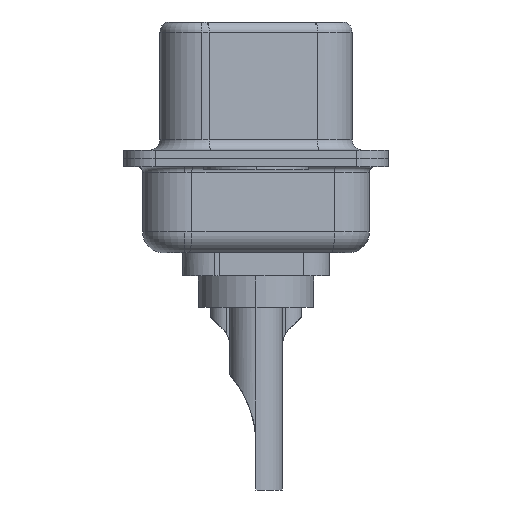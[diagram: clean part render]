
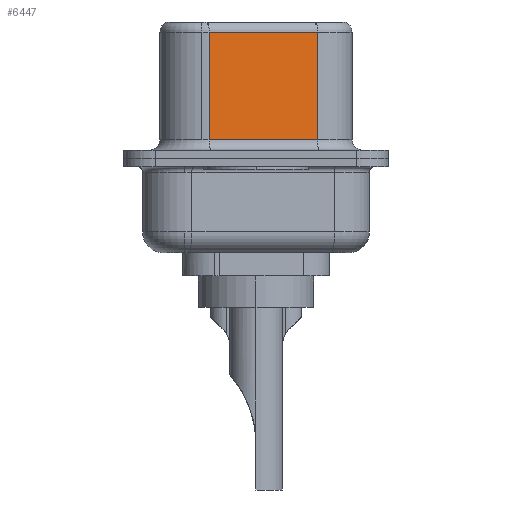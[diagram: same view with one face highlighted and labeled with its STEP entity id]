
A CAD part, left-side view. The second image highlights one B-rep face of the part: STEP entity #6447.
In plain terms, the highlighted planar face has unit normal (-0.985, -0.174, 0).
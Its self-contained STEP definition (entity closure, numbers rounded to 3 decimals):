
#517 = DIRECTION ( 'NONE',  ( 0.985, 0.174, 0. ) ) ;
#656 = DIRECTION ( 'NONE',  ( 0.174, -0.985, 0. ) ) ;
#715 = VECTOR ( 'NONE', #656, 1000. ) ;
#895 = EDGE_CURVE ( 'NONE', #2438, #12304, #14411, .T. ) ;
#1305 = AXIS2_PLACEMENT_3D ( 'NONE', #20225, #517, #16758 ) ;
#2438 = VERTEX_POINT ( 'NONE', #20954 ) ;
#2993 = CARTESIAN_POINT ( 'NONE',  ( 3.67, 2.233, 0.9 ) ) ;
#3220 = ORIENTED_EDGE ( 'NONE', *, *, #12690, .F. ) ;
#3221 = VERTEX_POINT ( 'NONE', #16325 ) ;
#3273 = VECTOR ( 'NONE', #15932, 1000. ) ;
#3303 = DIRECTION ( 'NONE',  ( -0.174, 0.985, 0. ) ) ;
#3773 = EDGE_CURVE ( 'NONE', #12304, #20291, #18393, .T. ) ;
#5034 = LINE ( 'NONE', #10408, #715 ) ;
#6155 = CARTESIAN_POINT ( 'NONE',  ( 4.58, -2.927, 6.52 ) ) ;
#6447 = ADVANCED_FACE ( 'NONE', ( #16624 ), #12303, .F. ) ;
#6517 = ORIENTED_EDGE ( 'NONE', *, *, #895, .T. ) ;
#9609 = ORIENTED_EDGE ( 'NONE', *, *, #3773, .T. ) ;
#9735 = VECTOR ( 'NONE', #19450, 1000. ) ;
#9785 = CARTESIAN_POINT ( 'NONE',  ( 3.67, 2.233, 6.02 ) ) ;
#9902 = ORIENTED_EDGE ( 'NONE', *, *, #18076, .T. ) ;
#10408 = CARTESIAN_POINT ( 'NONE',  ( 4.58, -2.927, 0.9 ) ) ;
#10554 = VECTOR ( 'NONE', #3303, 1000. ) ;
#11440 = LINE ( 'NONE', #6155, #3273 ) ;
#12303 = PLANE ( 'NONE',  #1305 ) ;
#12304 = VERTEX_POINT ( 'NONE', #9785 ) ;
#12690 = EDGE_CURVE ( 'NONE', #2438, #3221, #11440, .T. ) ;
#13580 = CARTESIAN_POINT ( 'NONE',  ( 4.58, -2.927, 6.02 ) ) ;
#13636 = CARTESIAN_POINT ( 'NONE',  ( 3.67, 2.233, 6.52 ) ) ;
#14411 = LINE ( 'NONE', #13580, #10554 ) ;
#15401 = EDGE_LOOP ( 'NONE', ( #3220, #6517, #9609, #9902 ) ) ;
#15932 = DIRECTION ( 'NONE',  ( 0., 0., -1. ) ) ;
#16325 = CARTESIAN_POINT ( 'NONE',  ( 4.58, -2.927, 0.9 ) ) ;
#16624 = FACE_OUTER_BOUND ( 'NONE', #15401, .T. ) ;
#16758 = DIRECTION ( 'NONE',  ( -0.174, 0.985, 0. ) ) ;
#18076 = EDGE_CURVE ( 'NONE', #20291, #3221, #5034, .T. ) ;
#18393 = LINE ( 'NONE', #13636, #9735 ) ;
#19450 = DIRECTION ( 'NONE',  ( 0., 0., -1. ) ) ;
#20225 = CARTESIAN_POINT ( 'NONE',  ( 4.58, -2.927, 6.52 ) ) ;
#20291 = VERTEX_POINT ( 'NONE', #2993 ) ;
#20954 = CARTESIAN_POINT ( 'NONE',  ( 4.58, -2.927, 6.02 ) ) ;
